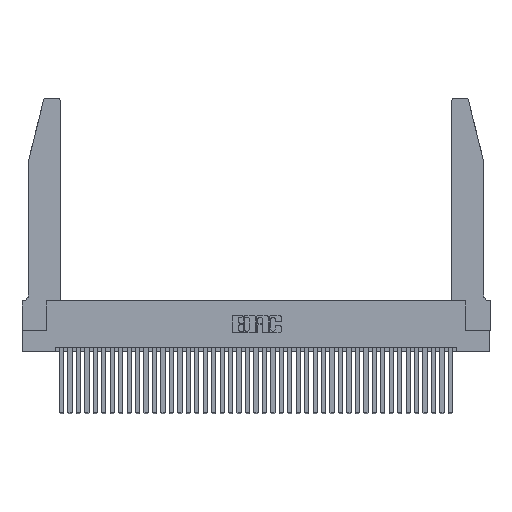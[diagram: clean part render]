
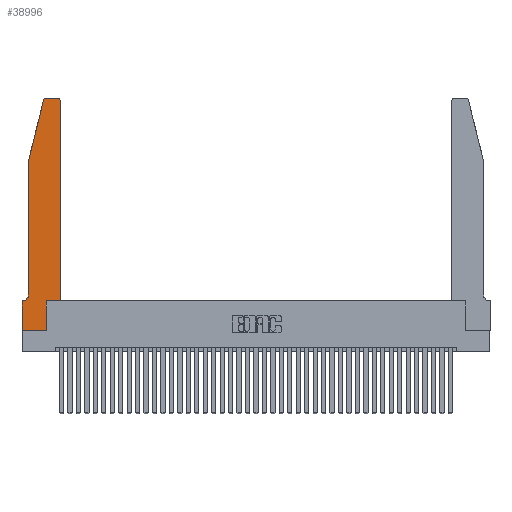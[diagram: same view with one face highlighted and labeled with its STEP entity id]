
A CAD part, top view. The second image highlights one B-rep face of the part: STEP entity #38996.
In plain terms, the highlighted planar face has unit normal (0, 0, 1).
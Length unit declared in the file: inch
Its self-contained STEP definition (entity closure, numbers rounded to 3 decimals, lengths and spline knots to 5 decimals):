
#1822 = CIRCLE ( 'NONE', #19758, 0.07 ) ;
#1902 = DIRECTION ( 'NONE',  ( -1., 0., 0. ) ) ;
#1982 = CARTESIAN_POINT ( 'NONE',  ( 0., 0., 0.37 ) ) ;
#2034 = ORIENTED_EDGE ( 'NONE', *, *, #34339, .T. ) ;
#2142 = CARTESIAN_POINT ( 'NONE',  ( 0.2865, 0.35, 0.37 ) ) ;
#2291 = ORIENTED_EDGE ( 'NONE', *, *, #33123, .T. ) ;
#3025 = VECTOR ( 'NONE', #15927, 39.37008 ) ;
#3458 = DIRECTION ( 'NONE',  ( -1., 0., 0. ) ) ;
#5463 = DIRECTION ( 'NONE',  ( 0., -1., 0. ) ) ;
#5567 = VERTEX_POINT ( 'NONE', #23556 ) ;
#5759 = VECTOR ( 'NONE', #5463, 39.37008 ) ;
#6026 = CARTESIAN_POINT ( 'NONE',  ( 0.0755, 2., 0.37 ) ) ;
#6253 = DIRECTION ( 'NONE',  ( 0., 0., 1. ) ) ;
#6357 = CARTESIAN_POINT ( 'NONE',  ( 0.284, 2.75, 0.37 ) ) ;
#6359 = VECTOR ( 'NONE', #30769, 39.37008 ) ;
#7073 = LINE ( 'NONE', #40459, #39612 ) ;
#7248 = CARTESIAN_POINT ( 'NONE',  ( 0.25487, 2.72718, 0.37 ) ) ;
#7491 = VECTOR ( 'NONE', #27987, 39.37008 ) ;
#8573 = CARTESIAN_POINT ( 'NONE',  ( 0.4505, 0.35, 0.37 ) ) ;
#8681 = DIRECTION ( 'NONE',  ( 0., 0., 1. ) ) ;
#8943 = CARTESIAN_POINT ( 'NONE',  ( 0.0055, 0.35, 0.37 ) ) ;
#9060 = CARTESIAN_POINT ( 'NONE',  ( 0.0755, 2., 0.37 ) ) ;
#9374 = AXIS2_PLACEMENT_3D ( 'NONE', #33201, #8681, #29871 ) ;
#9713 = DIRECTION ( 'NONE',  ( -0.239, -0.971, 0. ) ) ;
#11220 = EDGE_CURVE ( 'NONE', #28886, #40560, #35631, .T. ) ;
#11690 = EDGE_CURVE ( 'NONE', #12845, #13307, #7073, .T. ) ;
#11922 = DIRECTION ( 'NONE',  ( 1., 0., 0. ) ) ;
#12334 = DIRECTION ( 'NONE',  ( 0., 0., 1. ) ) ;
#12439 = CIRCLE ( 'NONE', #30792, 0.03 ) ;
#12607 = LINE ( 'NONE', #31879, #36263 ) ;
#12610 = DIRECTION ( 'NONE',  ( -1., 0., 0. ) ) ;
#12845 = VERTEX_POINT ( 'NONE', #7248 ) ;
#13136 = ORIENTED_EDGE ( 'NONE', *, *, #11690, .T. ) ;
#13307 = VERTEX_POINT ( 'NONE', #6026 ) ;
#13502 = CARTESIAN_POINT ( 'NONE',  ( 0., 0., 0.37 ) ) ;
#13537 = ORIENTED_EDGE ( 'NONE', *, *, #19056, .T. ) ;
#13693 = VERTEX_POINT ( 'NONE', #15815 ) ;
#13936 = VERTEX_POINT ( 'NONE', #29304 ) ;
#14147 = EDGE_CURVE ( 'NONE', #13307, #17198, #30873, .T. ) ;
#15815 = CARTESIAN_POINT ( 'NONE',  ( 0.4505, 2.72, 0.37 ) ) ;
#15927 = DIRECTION ( 'NONE',  ( 0., 1., 0. ) ) ;
#16268 = CARTESIAN_POINT ( 'NONE',  ( 0.2865, 0., 0.37 ) ) ;
#16296 = EDGE_CURVE ( 'NONE', #18815, #12845, #12439, .T. ) ;
#16586 = EDGE_CURVE ( 'NONE', #17254, #13936, #25754, .T. ) ;
#17198 = VERTEX_POINT ( 'NONE', #21002 ) ;
#17254 = VERTEX_POINT ( 'NONE', #16268 ) ;
#17327 = LINE ( 'NONE', #25416, #3025 ) ;
#18244 = ORIENTED_EDGE ( 'NONE', *, *, #11220, .T. ) ;
#18659 = DIRECTION ( 'NONE',  ( 0., -1., 0. ) ) ;
#18815 = VERTEX_POINT ( 'NONE', #6357 ) ;
#19056 = EDGE_CURVE ( 'NONE', #40560, #17254, #22614, .T. ) ;
#19138 = CIRCLE ( 'NONE', #9374, 0.03 ) ;
#19431 = ORIENTED_EDGE ( 'NONE', *, *, #16586, .T. ) ;
#19758 = AXIS2_PLACEMENT_3D ( 'NONE', #29072, #35408, #3458 ) ;
#21002 = CARTESIAN_POINT ( 'NONE',  ( 0.0755, 0.42, 0.37 ) ) ;
#21383 = CARTESIAN_POINT ( 'NONE',  ( 0.4505, 0.35, 0.37 ) ) ;
#22401 = DIRECTION ( 'NONE',  ( 1., 0., 0. ) ) ;
#22614 = LINE ( 'NONE', #1982, #6359 ) ;
#23464 = EDGE_CURVE ( 'NONE', #5567, #18815, #33937, .T. ) ;
#23556 = CARTESIAN_POINT ( 'NONE',  ( 0.4205, 2.75, 0.37 ) ) ;
#24591 = FACE_OUTER_BOUND ( 'NONE', #32257, .T. ) ;
#24890 = ORIENTED_EDGE ( 'NONE', *, *, #27945, .T. ) ;
#25416 = CARTESIAN_POINT ( 'NONE',  ( 0.4505, 0.35, 0.37 ) ) ;
#25528 = PLANE ( 'NONE',  #37822 ) ;
#25565 = VECTOR ( 'NONE', #1902, 39.37008 ) ;
#25754 = LINE ( 'NONE', #2142, #35568 ) ;
#26124 = ORIENTED_EDGE ( 'NONE', *, *, #23464, .T. ) ;
#27024 = EDGE_CURVE ( 'NONE', #13936, #29437, #31192, .T. ) ;
#27285 = VECTOR ( 'NONE', #18659, 39.37008 ) ;
#27945 = EDGE_CURVE ( 'NONE', #29437, #13693, #17327, .T. ) ;
#27987 = DIRECTION ( 'NONE',  ( 1., 0., 0. ) ) ;
#28886 = VERTEX_POINT ( 'NONE', #33851 ) ;
#29072 = CARTESIAN_POINT ( 'NONE',  ( 0.0055, 0.42, 0.37 ) ) ;
#29304 = CARTESIAN_POINT ( 'NONE',  ( 0.2865, 0.35, 0.37 ) ) ;
#29437 = VERTEX_POINT ( 'NONE', #8573 ) ;
#29871 = DIRECTION ( 'NONE',  ( 1., 0., 0. ) ) ;
#29887 = EDGE_CURVE ( 'NONE', #13693, #5567, #19138, .T. ) ;
#30769 = DIRECTION ( 'NONE',  ( 1., 0., 0. ) ) ;
#30792 = AXIS2_PLACEMENT_3D ( 'NONE', #31200, #12334, #11922 ) ;
#30873 = LINE ( 'NONE', #9060, #5759 ) ;
#31192 = LINE ( 'NONE', #21383, #7491 ) ;
#31200 = CARTESIAN_POINT ( 'NONE',  ( 0.284, 2.72, 0.37 ) ) ;
#31217 = DIRECTION ( 'NONE',  ( 0., 1., 0. ) ) ;
#31454 = CARTESIAN_POINT ( 'NONE',  ( 0., 0.35, 0.37 ) ) ;
#31752 = VERTEX_POINT ( 'NONE', #8943 ) ;
#31879 = CARTESIAN_POINT ( 'NONE',  ( 0.0755, 0.35, 0.37 ) ) ;
#32157 = ORIENTED_EDGE ( 'NONE', *, *, #16296, .T. ) ;
#32257 = EDGE_LOOP ( 'NONE', ( #26124, #32157, #13136, #39996, #2291, #2034, #18244, #13537, #19431, #39492, #24890, #36097 ) ) ;
#33123 = EDGE_CURVE ( 'NONE', #17198, #31752, #1822, .T. ) ;
#33201 = CARTESIAN_POINT ( 'NONE',  ( 0.4205, 2.72, 0.37 ) ) ;
#33851 = CARTESIAN_POINT ( 'NONE',  ( 0., 0.35, 0.37 ) ) ;
#33937 = LINE ( 'NONE', #39385, #25565 ) ;
#34339 = EDGE_CURVE ( 'NONE', #31752, #28886, #12607, .T. ) ;
#35408 = DIRECTION ( 'NONE',  ( 0., 0., -1. ) ) ;
#35568 = VECTOR ( 'NONE', #31217, 39.37008 ) ;
#35631 = LINE ( 'NONE', #37353, #27285 ) ;
#36097 = ORIENTED_EDGE ( 'NONE', *, *, #29887, .T. ) ;
#36263 = VECTOR ( 'NONE', #12610, 39.37008 ) ;
#37353 = CARTESIAN_POINT ( 'NONE',  ( 0., 0., 0.37 ) ) ;
#37822 = AXIS2_PLACEMENT_3D ( 'NONE', #31454, #6253, #22401 ) ;
#38996 = ADVANCED_FACE ( 'NONE', ( #24591 ), #25528, .T. ) ;
#39385 = CARTESIAN_POINT ( 'NONE',  ( 0.2605, 2.75, 0.37 ) ) ;
#39492 = ORIENTED_EDGE ( 'NONE', *, *, #27024, .T. ) ;
#39612 = VECTOR ( 'NONE', #9713, 39.37008 ) ;
#39996 = ORIENTED_EDGE ( 'NONE', *, *, #14147, .T. ) ;
#40459 = CARTESIAN_POINT ( 'NONE',  ( 0.0755, 2., 0.37 ) ) ;
#40560 = VERTEX_POINT ( 'NONE', #13502 ) ;
